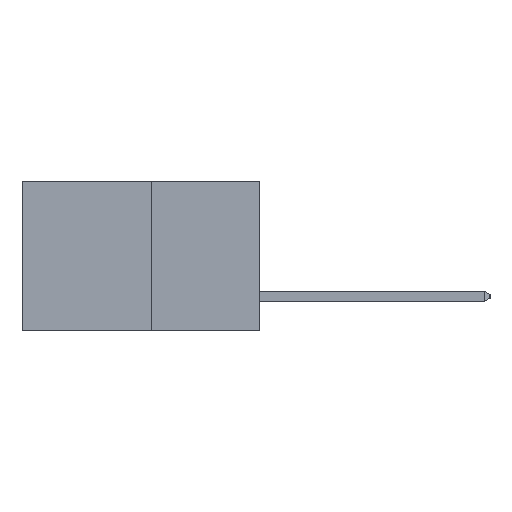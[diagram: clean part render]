
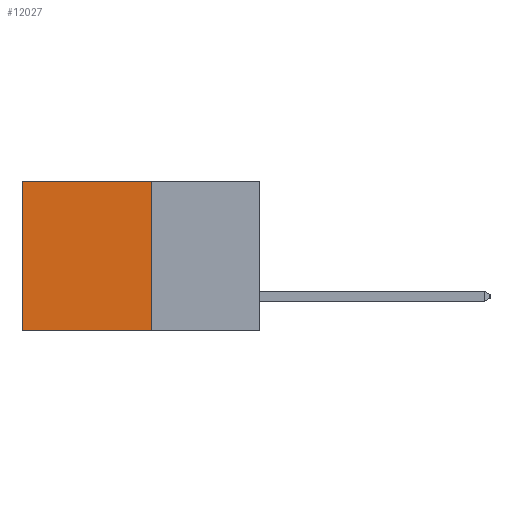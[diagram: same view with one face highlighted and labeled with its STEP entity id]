
A CAD part, left-side view. The second image highlights one B-rep face of the part: STEP entity #12027.
In plain terms, the highlighted planar face has unit normal (-1, 0, 0).
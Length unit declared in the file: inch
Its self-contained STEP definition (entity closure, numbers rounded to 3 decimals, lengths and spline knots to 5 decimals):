
#27 = ORIENTED_EDGE ( 'NONE', *, *, #1739, .F. ) ;
#45 = ORIENTED_EDGE ( 'NONE', *, *, #11782, .T. ) ;
#470 = LINE ( 'NONE', #11506, #5960 ) ;
#507 = DIRECTION ( 'NONE',  ( 0., 0., -1. ) ) ;
#799 = EDGE_LOOP ( 'NONE', ( #45, #27, #3586, #1014 ) ) ;
#965 = CARTESIAN_POINT ( 'NONE',  ( 0.277, 0.27, -0.37 ) ) ;
#1014 = ORIENTED_EDGE ( 'NONE', *, *, #9266, .T. ) ;
#1739 = EDGE_CURVE ( 'NONE', #2232, #10304, #5537, .T. ) ;
#1806 = LINE ( 'NONE', #965, #4375 ) ;
#1836 = VECTOR ( 'NONE', #507, 39.37008 ) ;
#2232 = VERTEX_POINT ( 'NONE', #11772 ) ;
#2326 = VECTOR ( 'NONE', #13586, 39.37008 ) ;
#3210 = VERTEX_POINT ( 'NONE', #3558 ) ;
#3558 = CARTESIAN_POINT ( 'NONE',  ( 0.277, 0.59, 0. ) ) ;
#3586 = ORIENTED_EDGE ( 'NONE', *, *, #13168, .F. ) ;
#3912 = VERTEX_POINT ( 'NONE', #13103 ) ;
#4375 = VECTOR ( 'NONE', #13488, 39.37008 ) ;
#5356 = CARTESIAN_POINT ( 'NONE',  ( 0.277, 0.27, -0.37 ) ) ;
#5537 = LINE ( 'NONE', #6914, #2326 ) ;
#5960 = VECTOR ( 'NONE', #7458, 39.37008 ) ;
#6439 = DIRECTION ( 'NONE',  ( 0., 0., -1. ) ) ;
#6914 = CARTESIAN_POINT ( 'NONE',  ( 0.277, 0.27, -0.37 ) ) ;
#7064 = CARTESIAN_POINT ( 'NONE',  ( 0.277, 0.59, -0.37 ) ) ;
#7458 = DIRECTION ( 'NONE',  ( 0., 1., 0. ) ) ;
#9266 = EDGE_CURVE ( 'NONE', #3912, #3210, #470, .T. ) ;
#9856 = AXIS2_PLACEMENT_3D ( 'NONE', #5356, #12547, #6439 ) ;
#10304 = VERTEX_POINT ( 'NONE', #12089 ) ;
#11506 = CARTESIAN_POINT ( 'NONE',  ( 0.277, 0.27, 0. ) ) ;
#11560 = PLANE ( 'NONE',  #9856 ) ;
#11709 = LINE ( 'NONE', #7064, #1836 ) ;
#11772 = CARTESIAN_POINT ( 'NONE',  ( 0.277, 0.27, -0.37 ) ) ;
#11782 = EDGE_CURVE ( 'NONE', #3210, #10304, #11709, .T. ) ;
#12027 = ADVANCED_FACE ( 'NONE', ( #13525 ), #11560, .F. ) ;
#12089 = CARTESIAN_POINT ( 'NONE',  ( 0.277, 0.59, -0.37 ) ) ;
#12547 = DIRECTION ( 'NONE',  ( 1., 0., 0. ) ) ;
#13103 = CARTESIAN_POINT ( 'NONE',  ( 0.277, 0.27, 0. ) ) ;
#13168 = EDGE_CURVE ( 'NONE', #3912, #2232, #1806, .T. ) ;
#13488 = DIRECTION ( 'NONE',  ( 0., 0., -1. ) ) ;
#13525 = FACE_OUTER_BOUND ( 'NONE', #799, .T. ) ;
#13586 = DIRECTION ( 'NONE',  ( 0., 1., 0. ) ) ;
